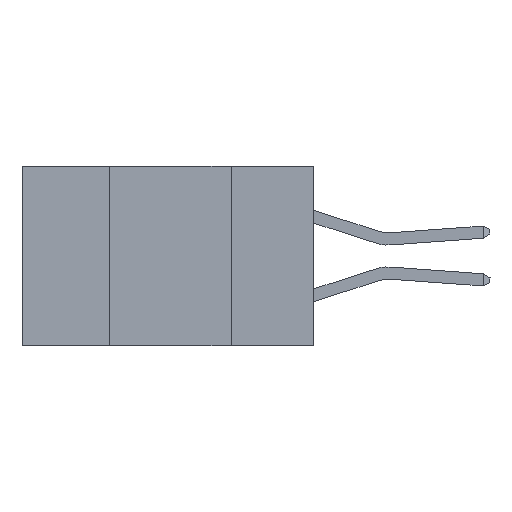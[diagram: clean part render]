
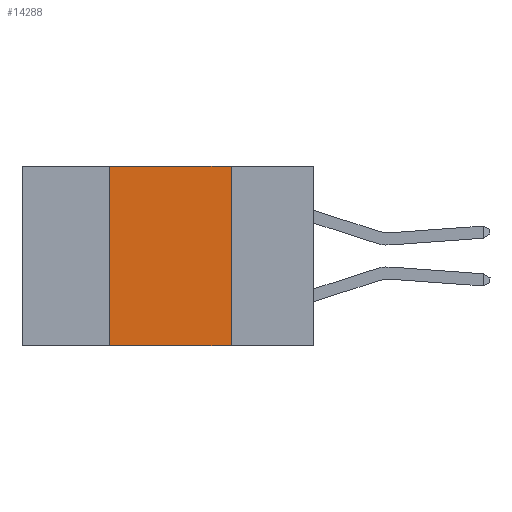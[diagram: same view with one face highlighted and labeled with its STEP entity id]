
A CAD part, left-side view. The second image highlights one B-rep face of the part: STEP entity #14288.
In plain terms, the highlighted planar face has unit normal (-1, 0, 0).
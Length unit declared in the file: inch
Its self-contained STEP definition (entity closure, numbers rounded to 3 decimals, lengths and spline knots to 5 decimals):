
#476 = EDGE_CURVE ( 'NONE', #5499, #18272, #9697, .T. ) ;
#697 = EDGE_CURVE ( 'NONE', #18272, #10053, #4201, .T. ) ;
#972 = FACE_OUTER_BOUND ( 'NONE', #14581, .T. ) ;
#1754 = VECTOR ( 'NONE', #23781, 39.37008 ) ;
#2120 = AXIS2_PLACEMENT_3D ( 'NONE', #17032, #22915, #20666 ) ;
#4019 = CARTESIAN_POINT ( 'NONE',  ( 0., 0.6, -0.37 ) ) ;
#4201 = LINE ( 'NONE', #12176, #14701 ) ;
#4531 = ORIENTED_EDGE ( 'NONE', *, *, #697, .F. ) ;
#4642 = CARTESIAN_POINT ( 'NONE',  ( 0., 0.17, 0. ) ) ;
#5499 = VERTEX_POINT ( 'NONE', #5935 ) ;
#5935 = CARTESIAN_POINT ( 'NONE',  ( 0., 0.42, -0.37 ) ) ;
#6284 = ORIENTED_EDGE ( 'NONE', *, *, #476, .F. ) ;
#6344 = DIRECTION ( 'NONE',  ( 0., 0., -1. ) ) ;
#8927 = PLANE ( 'NONE',  #2120 ) ;
#9697 = LINE ( 'NONE', #9936, #20116 ) ;
#9859 = ORIENTED_EDGE ( 'NONE', *, *, #15217, .T. ) ;
#9936 = CARTESIAN_POINT ( 'NONE',  ( 0., 0.42, 0. ) ) ;
#10053 = VERTEX_POINT ( 'NONE', #16159 ) ;
#12176 = CARTESIAN_POINT ( 'NONE',  ( 0., 0.6, 0. ) ) ;
#14288 = ADVANCED_FACE ( 'NONE', ( #972 ), #8927, .F. ) ;
#14429 = CARTESIAN_POINT ( 'NONE',  ( 0., 0.17, -0.37 ) ) ;
#14576 = LINE ( 'NONE', #4642, #20401 ) ;
#14581 = EDGE_LOOP ( 'NONE', ( #15699, #4531, #6284, #9859 ) ) ;
#14701 = VECTOR ( 'NONE', #18170, 39.37008 ) ;
#15217 = EDGE_CURVE ( 'NONE', #5499, #18992, #17626, .T. ) ;
#15699 = ORIENTED_EDGE ( 'NONE', *, *, #20257, .F. ) ;
#16159 = CARTESIAN_POINT ( 'NONE',  ( 0., 0.17, 0. ) ) ;
#17032 = CARTESIAN_POINT ( 'NONE',  ( 0., 0.6, 0. ) ) ;
#17626 = LINE ( 'NONE', #4019, #1754 ) ;
#18170 = DIRECTION ( 'NONE',  ( 0., -1., 0. ) ) ;
#18272 = VERTEX_POINT ( 'NONE', #20753 ) ;
#18992 = VERTEX_POINT ( 'NONE', #14429 ) ;
#20116 = VECTOR ( 'NONE', #21327, 39.37008 ) ;
#20257 = EDGE_CURVE ( 'NONE', #10053, #18992, #14576, .T. ) ;
#20401 = VECTOR ( 'NONE', #6344, 39.37008 ) ;
#20666 = DIRECTION ( 'NONE',  ( 0., 0., -1. ) ) ;
#20753 = CARTESIAN_POINT ( 'NONE',  ( 0., 0.42, 0. ) ) ;
#21327 = DIRECTION ( 'NONE',  ( 0., 0., 1. ) ) ;
#22915 = DIRECTION ( 'NONE',  ( 1., 0., 0. ) ) ;
#23781 = DIRECTION ( 'NONE',  ( 0., -1., 0. ) ) ;
